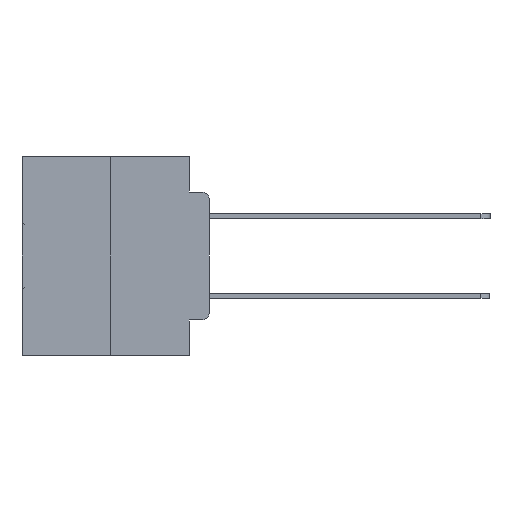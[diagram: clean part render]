
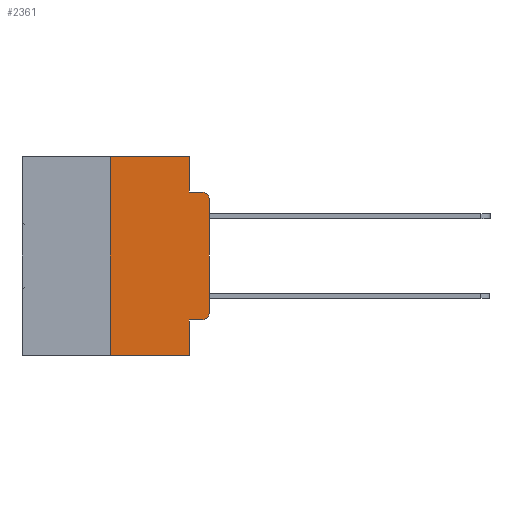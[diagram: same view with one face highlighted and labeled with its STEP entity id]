
A CAD part, left-side view. The second image highlights one B-rep face of the part: STEP entity #2361.
In plain terms, the highlighted planar face has unit normal (-1, 0, 0).
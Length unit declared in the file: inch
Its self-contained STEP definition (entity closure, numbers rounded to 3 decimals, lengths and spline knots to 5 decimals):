
#164 = CARTESIAN_POINT ( 'NONE',  ( 0., 0.473, 0. ) ) ;
#313 = CARTESIAN_POINT ( 'NONE',  ( 0., 0.25, 0. ) ) ;
#532 = DIRECTION ( 'NONE',  ( 0., 0., -1. ) ) ;
#896 = CARTESIAN_POINT ( 'NONE',  ( 0., 0.051, -0.5 ) ) ;
#1633 = LINE ( 'NONE', #164, #28127 ) ;
#2022 = VECTOR ( 'NONE', #17546, 39.37008 ) ;
#2361 = ADVANCED_FACE ( 'NONE', ( #13432 ), #24358, .F. ) ;
#2630 = LINE ( 'NONE', #18681, #29121 ) ;
#2667 = CARTESIAN_POINT ( 'NONE',  ( 0., 0., -0.1085 ) ) ;
#3115 = CARTESIAN_POINT ( 'NONE',  ( 0., 0.051, -0.0885 ) ) ;
#3986 = CARTESIAN_POINT ( 'NONE',  ( 0., 0.25, 0. ) ) ;
#4088 = VECTOR ( 'NONE', #29915, 39.37008 ) ;
#4146 = ORIENTED_EDGE ( 'NONE', *, *, #16776, .T. ) ;
#4249 = CARTESIAN_POINT ( 'NONE',  ( 0., 0.473, -0.5 ) ) ;
#4896 = CARTESIAN_POINT ( 'NONE',  ( 0., 0.051, -0.4115 ) ) ;
#4913 = ORIENTED_EDGE ( 'NONE', *, *, #10390, .F. ) ;
#5008 = EDGE_CURVE ( 'NONE', #30275, #20143, #1633, .T. ) ;
#6283 = CARTESIAN_POINT ( 'NONE',  ( 0., 0.051, 0. ) ) ;
#6762 = CARTESIAN_POINT ( 'NONE',  ( 0., 0.051, 0. ) ) ;
#7319 = EDGE_CURVE ( 'NONE', #20143, #25949, #22156, .T. ) ;
#7454 = VERTEX_POINT ( 'NONE', #9964 ) ;
#8030 = VERTEX_POINT ( 'NONE', #29573 ) ;
#8276 = ORIENTED_EDGE ( 'NONE', *, *, #12712, .T. ) ;
#9196 = CARTESIAN_POINT ( 'NONE',  ( 0., 0.02, -0.3915 ) ) ;
#9762 = CIRCLE ( 'NONE', #12219, 0.02 ) ;
#9964 = CARTESIAN_POINT ( 'NONE',  ( 0., 0.02, -0.0885 ) ) ;
#10222 = VERTEX_POINT ( 'NONE', #14357 ) ;
#10390 = EDGE_CURVE ( 'NONE', #10222, #13611, #2630, .T. ) ;
#10543 = ORIENTED_EDGE ( 'NONE', *, *, #19825, .T. ) ;
#10793 = CARTESIAN_POINT ( 'NONE',  ( 0., 0.02, -0.1085 ) ) ;
#11773 = DIRECTION ( 'NONE',  ( 0., 0., -1. ) ) ;
#12219 = AXIS2_PLACEMENT_3D ( 'NONE', #10793, #28661, #13316 ) ;
#12536 = EDGE_CURVE ( 'NONE', #28999, #13611, #24570, .T. ) ;
#12712 = EDGE_CURVE ( 'NONE', #10222, #16331, #32431, .T. ) ;
#12904 = LINE ( 'NONE', #3986, #25726 ) ;
#13152 = EDGE_CURVE ( 'NONE', #28999, #30275, #12904, .T. ) ;
#13235 = CARTESIAN_POINT ( 'NONE',  ( 0., 0.25, -0.5 ) ) ;
#13316 = DIRECTION ( 'NONE',  ( 0., 0., -1. ) ) ;
#13432 = FACE_OUTER_BOUND ( 'NONE', #29276, .T. ) ;
#13611 = VERTEX_POINT ( 'NONE', #896 ) ;
#14357 = CARTESIAN_POINT ( 'NONE',  ( 0., 0.051, -0.4115 ) ) ;
#14536 = DIRECTION ( 'NONE',  ( 0., 0., -1. ) ) ;
#14558 = VERTEX_POINT ( 'NONE', #2667 ) ;
#14903 = LINE ( 'NONE', #3115, #20923 ) ;
#15115 = AXIS2_PLACEMENT_3D ( 'NONE', #32744, #22511, #22659 ) ;
#15711 = LINE ( 'NONE', #25160, #2022 ) ;
#16108 = VECTOR ( 'NONE', #14536, 39.37008 ) ;
#16331 = VERTEX_POINT ( 'NONE', #30106 ) ;
#16420 = DIRECTION ( 'NONE',  ( 0., -1., 0. ) ) ;
#16776 = EDGE_CURVE ( 'NONE', #16331, #8030, #29507, .T. ) ;
#16794 = DIRECTION ( 'NONE',  ( 0., 0., 1. ) ) ;
#17546 = DIRECTION ( 'NONE',  ( 0., 0., 1. ) ) ;
#18681 = CARTESIAN_POINT ( 'NONE',  ( 0., 0.051, 0. ) ) ;
#19825 = EDGE_CURVE ( 'NONE', #14558, #7454, #9762, .T. ) ;
#20143 = VERTEX_POINT ( 'NONE', #6762 ) ;
#20270 = EDGE_CURVE ( 'NONE', #8030, #14558, #15711, .T. ) ;
#20923 = VECTOR ( 'NONE', #31175, 39.37008 ) ;
#20970 = AXIS2_PLACEMENT_3D ( 'NONE', #9196, #27103, #11773 ) ;
#21787 = ORIENTED_EDGE ( 'NONE', *, *, #29032, .F. ) ;
#22156 = LINE ( 'NONE', #6283, #16108 ) ;
#22234 = ORIENTED_EDGE ( 'NONE', *, *, #7319, .F. ) ;
#22511 = DIRECTION ( 'NONE',  ( 1., 0., 0. ) ) ;
#22547 = ORIENTED_EDGE ( 'NONE', *, *, #20270, .T. ) ;
#22659 = DIRECTION ( 'NONE',  ( 0., 0., -1. ) ) ;
#23109 = ORIENTED_EDGE ( 'NONE', *, *, #13152, .F. ) ;
#24358 = PLANE ( 'NONE',  #15115 ) ;
#24570 = LINE ( 'NONE', #4249, #4088 ) ;
#25160 = CARTESIAN_POINT ( 'NONE',  ( 0., 0., 0. ) ) ;
#25334 = DIRECTION ( 'NONE',  ( 0., -1., 0. ) ) ;
#25726 = VECTOR ( 'NONE', #16794, 39.37008 ) ;
#25755 = VECTOR ( 'NONE', #25334, 39.37008 ) ;
#25949 = VERTEX_POINT ( 'NONE', #27720 ) ;
#27103 = DIRECTION ( 'NONE',  ( -1., 0., 0. ) ) ;
#27720 = CARTESIAN_POINT ( 'NONE',  ( 0., 0.051, -0.0885 ) ) ;
#28127 = VECTOR ( 'NONE', #16420, 39.37008 ) ;
#28271 = ORIENTED_EDGE ( 'NONE', *, *, #5008, .F. ) ;
#28661 = DIRECTION ( 'NONE',  ( -1., 0., 0. ) ) ;
#28999 = VERTEX_POINT ( 'NONE', #13235 ) ;
#29032 = EDGE_CURVE ( 'NONE', #25949, #7454, #14903, .T. ) ;
#29121 = VECTOR ( 'NONE', #532, 39.37008 ) ;
#29276 = EDGE_LOOP ( 'NONE', ( #22547, #10543, #21787, #22234, #28271, #23109, #30242, #4913, #8276, #4146 ) ) ;
#29507 = CIRCLE ( 'NONE', #20970, 0.02 ) ;
#29573 = CARTESIAN_POINT ( 'NONE',  ( 0., 0., -0.3915 ) ) ;
#29915 = DIRECTION ( 'NONE',  ( 0., -1., 0. ) ) ;
#30106 = CARTESIAN_POINT ( 'NONE',  ( 0., 0.02, -0.4115 ) ) ;
#30242 = ORIENTED_EDGE ( 'NONE', *, *, #12536, .T. ) ;
#30275 = VERTEX_POINT ( 'NONE', #313 ) ;
#31175 = DIRECTION ( 'NONE',  ( 0., -1., 0. ) ) ;
#32431 = LINE ( 'NONE', #4896, #25755 ) ;
#32744 = CARTESIAN_POINT ( 'NONE',  ( 0., 0.473, 0. ) ) ;
